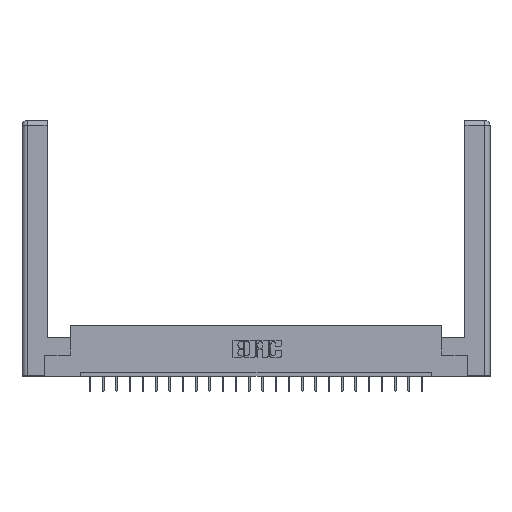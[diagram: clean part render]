
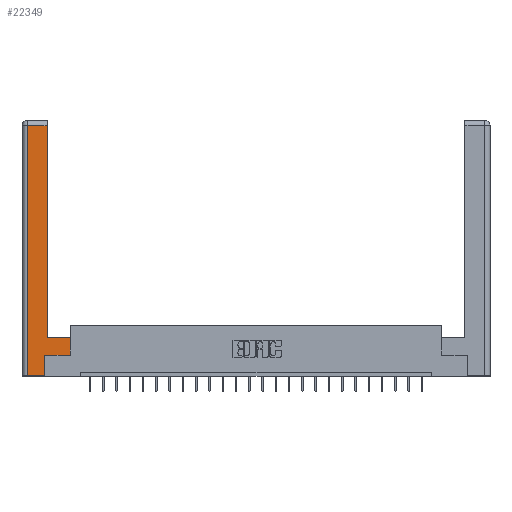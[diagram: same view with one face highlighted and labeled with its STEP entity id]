
A CAD part, top view. The second image highlights one B-rep face of the part: STEP entity #22349.
In plain terms, the highlighted planar face has unit normal (0, 0, 1).
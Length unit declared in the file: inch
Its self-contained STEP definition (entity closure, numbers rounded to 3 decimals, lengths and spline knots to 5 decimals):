
#95 = VECTOR ( 'NONE', #19705, 39.37008 ) ;
#191 = ORIENTED_EDGE ( 'NONE', *, *, #23261, .T. ) ;
#540 = DIRECTION ( 'NONE',  ( 0., 1., 0. ) ) ;
#704 = CARTESIAN_POINT ( 'NONE',  ( 0.565, 0.45, 0. ) ) ;
#1043 = VERTEX_POINT ( 'NONE', #13319 ) ;
#1095 = CARTESIAN_POINT ( 'NONE',  ( 0.565, 0.45, 0. ) ) ;
#2690 = DIRECTION ( 'NONE',  ( -1., 0., 0. ) ) ;
#2816 = AXIS2_PLACEMENT_3D ( 'NONE', #17512, #21243, #23143 ) ;
#3175 = EDGE_LOOP ( 'NONE', ( #7556, #4257, #4719, #191, #23315, #19433, #22941, #14101 ) ) ;
#3394 = VECTOR ( 'NONE', #23010, 39.37008 ) ;
#3712 = CARTESIAN_POINT ( 'NONE',  ( 0.0615, 0., 0. ) ) ;
#4257 = ORIENTED_EDGE ( 'NONE', *, *, #14904, .T. ) ;
#4416 = LINE ( 'NONE', #11884, #23653 ) ;
#4529 = VECTOR ( 'NONE', #23338, 39.37008 ) ;
#4550 = CARTESIAN_POINT ( 'NONE',  ( 0.265, 0.245, 0. ) ) ;
#4688 = VECTOR ( 'NONE', #11293, 39.37008 ) ;
#4696 = LINE ( 'NONE', #20320, #19791 ) ;
#4719 = ORIENTED_EDGE ( 'NONE', *, *, #22036, .T. ) ;
#5121 = CARTESIAN_POINT ( 'NONE',  ( 0.0615, 2.94, 0. ) ) ;
#5448 = CARTESIAN_POINT ( 'NONE',  ( 0.265, 0.245, 0. ) ) ;
#5618 = DIRECTION ( 'NONE',  ( 1., 0., 0. ) ) ;
#6116 = VECTOR ( 'NONE', #540, 39.37008 ) ;
#6244 = EDGE_CURVE ( 'NONE', #8198, #16275, #19364, .T. ) ;
#7184 = CARTESIAN_POINT ( 'NONE',  ( 0.295, 2.94, 0. ) ) ;
#7378 = CARTESIAN_POINT ( 'NONE',  ( 0.265, 0., 0. ) ) ;
#7556 = ORIENTED_EDGE ( 'NONE', *, *, #20995, .T. ) ;
#8198 = VERTEX_POINT ( 'NONE', #23279 ) ;
#8305 = CARTESIAN_POINT ( 'NONE',  ( 0.0615, 2.94, 0. ) ) ;
#9983 = LINE ( 'NONE', #8305, #4529 ) ;
#10004 = EDGE_CURVE ( 'NONE', #16275, #1043, #4696, .T. ) ;
#10177 = CARTESIAN_POINT ( 'NONE',  ( 0.0615, 0., 0. ) ) ;
#10345 = VERTEX_POINT ( 'NONE', #7184 ) ;
#11293 = DIRECTION ( 'NONE',  ( 0., -1., 0. ) ) ;
#11884 = CARTESIAN_POINT ( 'NONE',  ( 0.295, 0.45, 0. ) ) ;
#12771 = LINE ( 'NONE', #3712, #4688 ) ;
#13319 = CARTESIAN_POINT ( 'NONE',  ( 0.565, 0.245, 0. ) ) ;
#14101 = ORIENTED_EDGE ( 'NONE', *, *, #21670, .T. ) ;
#14287 = VERTEX_POINT ( 'NONE', #1095 ) ;
#14544 = LINE ( 'NONE', #704, #6116 ) ;
#14609 = LINE ( 'NONE', #18117, #95 ) ;
#14904 = EDGE_CURVE ( 'NONE', #10345, #18302, #9983, .T. ) ;
#16275 = VERTEX_POINT ( 'NONE', #5448 ) ;
#17512 = CARTESIAN_POINT ( 'NONE',  ( 0., 0., 0. ) ) ;
#18117 = CARTESIAN_POINT ( 'NONE',  ( 0.295, 3., 0. ) ) ;
#18136 = VERTEX_POINT ( 'NONE', #10177 ) ;
#18302 = VERTEX_POINT ( 'NONE', #5121 ) ;
#18532 = DIRECTION ( 'NONE',  ( 1., 0., 0. ) ) ;
#19364 = LINE ( 'NONE', #4550, #3394 ) ;
#19433 = ORIENTED_EDGE ( 'NONE', *, *, #10004, .T. ) ;
#19453 = CARTESIAN_POINT ( 'NONE',  ( 0.295, 0.45, 0. ) ) ;
#19705 = DIRECTION ( 'NONE',  ( 0., 1., 0. ) ) ;
#19791 = VECTOR ( 'NONE', #18532, 39.37008 ) ;
#20320 = CARTESIAN_POINT ( 'NONE',  ( 0.565, 0.245, 0. ) ) ;
#20557 = LINE ( 'NONE', #7378, #21147 ) ;
#20995 = EDGE_CURVE ( 'NONE', #22408, #10345, #14609, .T. ) ;
#21147 = VECTOR ( 'NONE', #5618, 39.37008 ) ;
#21243 = DIRECTION ( 'NONE',  ( 0., 0., -1. ) ) ;
#21670 = EDGE_CURVE ( 'NONE', #14287, #22408, #4416, .T. ) ;
#22036 = EDGE_CURVE ( 'NONE', #18302, #18136, #12771, .T. ) ;
#22246 = EDGE_CURVE ( 'NONE', #1043, #14287, #14544, .T. ) ;
#22349 = ADVANCED_FACE ( 'NONE', ( #23604 ), #23406, .F. ) ;
#22408 = VERTEX_POINT ( 'NONE', #19453 ) ;
#22941 = ORIENTED_EDGE ( 'NONE', *, *, #22246, .T. ) ;
#23010 = DIRECTION ( 'NONE',  ( 0., 1., 0. ) ) ;
#23143 = DIRECTION ( 'NONE',  ( -1., 0., 0. ) ) ;
#23261 = EDGE_CURVE ( 'NONE', #18136, #8198, #20557, .T. ) ;
#23279 = CARTESIAN_POINT ( 'NONE',  ( 0.265, 0., 0. ) ) ;
#23315 = ORIENTED_EDGE ( 'NONE', *, *, #6244, .T. ) ;
#23338 = DIRECTION ( 'NONE',  ( -1., 0., 0. ) ) ;
#23406 = PLANE ( 'NONE',  #2816 ) ;
#23604 = FACE_OUTER_BOUND ( 'NONE', #3175, .T. ) ;
#23653 = VECTOR ( 'NONE', #2690, 39.37008 ) ;
